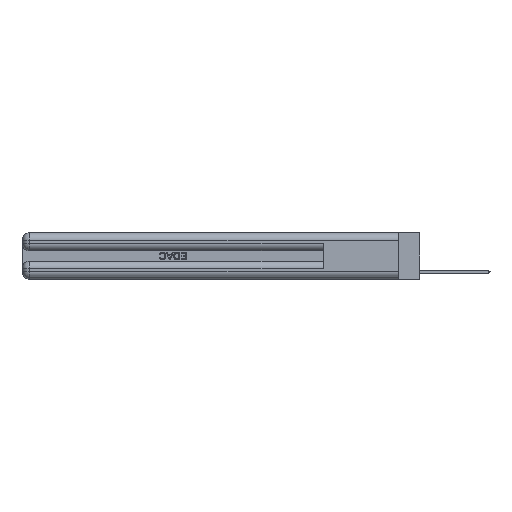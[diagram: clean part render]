
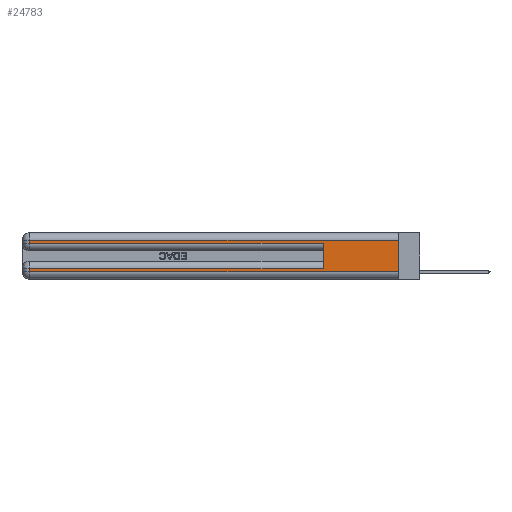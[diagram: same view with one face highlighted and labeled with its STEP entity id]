
A CAD part, left-side view. The second image highlights one B-rep face of the part: STEP entity #24783.
In plain terms, the highlighted planar face has unit normal (-1, 0, 0).
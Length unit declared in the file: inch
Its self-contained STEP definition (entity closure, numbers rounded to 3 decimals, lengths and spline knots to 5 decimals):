
#176 = CARTESIAN_POINT ( 'NONE',  ( 0., 2.94, 0.31 ) ) ;
#221 = CARTESIAN_POINT ( 'NONE',  ( 0., 0., 0.285 ) ) ;
#264 = VERTEX_POINT ( 'NONE', #13702 ) ;
#1384 = DIRECTION ( 'NONE',  ( 0., 1., 0. ) ) ;
#1541 = VECTOR ( 'NONE', #27089, 39.37008 ) ;
#1990 = CARTESIAN_POINT ( 'NONE',  ( 0., 2.94, 0.37 ) ) ;
#2046 = CARTESIAN_POINT ( 'NONE',  ( 0., 0., 0.085 ) ) ;
#2128 = VERTEX_POINT ( 'NONE', #9531 ) ;
#2401 = ORIENTED_EDGE ( 'NONE', *, *, #19415, .F. ) ;
#2549 = CARTESIAN_POINT ( 'NONE',  ( 0., 0., 0.37 ) ) ;
#2701 = CARTESIAN_POINT ( 'NONE',  ( 0., 0., 0.37 ) ) ;
#2798 = EDGE_CURVE ( 'NONE', #4129, #6630, #25447, .T. ) ;
#3160 = EDGE_CURVE ( 'NONE', #2128, #16401, #15424, .T. ) ;
#4129 = VERTEX_POINT ( 'NONE', #27358 ) ;
#5038 = PLANE ( 'NONE',  #22201 ) ;
#5551 = ORIENTED_EDGE ( 'NONE', *, *, #2798, .T. ) ;
#6630 = VERTEX_POINT ( 'NONE', #176 ) ;
#7138 = EDGE_LOOP ( 'NONE', ( #2401, #5551, #13132, #22939, #7952, #16491, #28968, #22165 ) ) ;
#7541 = FACE_OUTER_BOUND ( 'NONE', #7138, .T. ) ;
#7952 = ORIENTED_EDGE ( 'NONE', *, *, #21764, .F. ) ;
#8078 = DIRECTION ( 'NONE',  ( 1., 0., 0. ) ) ;
#8620 = DIRECTION ( 'NONE',  ( 0., -1., 0. ) ) ;
#9430 = CARTESIAN_POINT ( 'NONE',  ( 0., 2.94, 0.06 ) ) ;
#9531 = CARTESIAN_POINT ( 'NONE',  ( 0., 2.94, 0.085 ) ) ;
#9844 = CARTESIAN_POINT ( 'NONE',  ( 0., 2.94, 0.285 ) ) ;
#10744 = DIRECTION ( 'NONE',  ( 0., 0., -1. ) ) ;
#11096 = DIRECTION ( 'NONE',  ( 0., -1., 0. ) ) ;
#11472 = CARTESIAN_POINT ( 'NONE',  ( 0., 0., 0.06 ) ) ;
#12965 = CARTESIAN_POINT ( 'NONE',  ( 0., 0.6, 0.285 ) ) ;
#13132 = ORIENTED_EDGE ( 'NONE', *, *, #33599, .T. ) ;
#13702 = CARTESIAN_POINT ( 'NONE',  ( 0., 0.6, 0.085 ) ) ;
#14164 = VECTOR ( 'NONE', #20791, 39.37008 ) ;
#14275 = VECTOR ( 'NONE', #8620, 39.37008 ) ;
#14638 = EDGE_CURVE ( 'NONE', #19195, #33156, #25165, .T. ) ;
#15424 = LINE ( 'NONE', #15953, #23659 ) ;
#15442 = LINE ( 'NONE', #29126, #30635 ) ;
#15616 = LINE ( 'NONE', #2046, #14164 ) ;
#15953 = CARTESIAN_POINT ( 'NONE',  ( 0., 2.94, 0.37 ) ) ;
#16401 = VERTEX_POINT ( 'NONE', #9430 ) ;
#16491 = ORIENTED_EDGE ( 'NONE', *, *, #21850, .T. ) ;
#16903 = VECTOR ( 'NONE', #1384, 39.37008 ) ;
#18955 = DIRECTION ( 'NONE',  ( 0., 0., -1. ) ) ;
#19195 = VERTEX_POINT ( 'NONE', #9844 ) ;
#19415 = EDGE_CURVE ( 'NONE', #4129, #29878, #29768, .T. ) ;
#20791 = DIRECTION ( 'NONE',  ( 0., 1., 0. ) ) ;
#21601 = LINE ( 'NONE', #1990, #34695 ) ;
#21764 = EDGE_CURVE ( 'NONE', #264, #33156, #15442, .T. ) ;
#21850 = EDGE_CURVE ( 'NONE', #264, #2128, #15616, .T. ) ;
#22165 = ORIENTED_EDGE ( 'NONE', *, *, #22965, .T. ) ;
#22201 = AXIS2_PLACEMENT_3D ( 'NONE', #2549, #8078, #10744 ) ;
#22939 = ORIENTED_EDGE ( 'NONE', *, *, #14638, .T. ) ;
#22965 = EDGE_CURVE ( 'NONE', #16401, #29878, #30335, .T. ) ;
#23453 = DIRECTION ( 'NONE',  ( 0., 0., 1. ) ) ;
#23594 = VECTOR ( 'NONE', #11096, 39.37008 ) ;
#23659 = VECTOR ( 'NONE', #34307, 39.37008 ) ;
#24783 = ADVANCED_FACE ( 'NONE', ( #7541 ), #5038, .F. ) ;
#25165 = LINE ( 'NONE', #221, #23594 ) ;
#25447 = LINE ( 'NONE', #25793, #16903 ) ;
#25793 = CARTESIAN_POINT ( 'NONE',  ( 0., 0., 0.31 ) ) ;
#27089 = DIRECTION ( 'NONE',  ( 0., 0., -1. ) ) ;
#27358 = CARTESIAN_POINT ( 'NONE',  ( 0., 0., 0.31 ) ) ;
#28968 = ORIENTED_EDGE ( 'NONE', *, *, #3160, .T. ) ;
#29126 = CARTESIAN_POINT ( 'NONE',  ( 0., 0.6, 0.145 ) ) ;
#29768 = LINE ( 'NONE', #2701, #1541 ) ;
#29878 = VERTEX_POINT ( 'NONE', #30941 ) ;
#30335 = LINE ( 'NONE', #11472, #14275 ) ;
#30635 = VECTOR ( 'NONE', #23453, 39.37008 ) ;
#30941 = CARTESIAN_POINT ( 'NONE',  ( 0., 0., 0.06 ) ) ;
#33156 = VERTEX_POINT ( 'NONE', #12965 ) ;
#33599 = EDGE_CURVE ( 'NONE', #6630, #19195, #21601, .T. ) ;
#34307 = DIRECTION ( 'NONE',  ( 0., 0., -1. ) ) ;
#34695 = VECTOR ( 'NONE', #18955, 39.37008 ) ;
